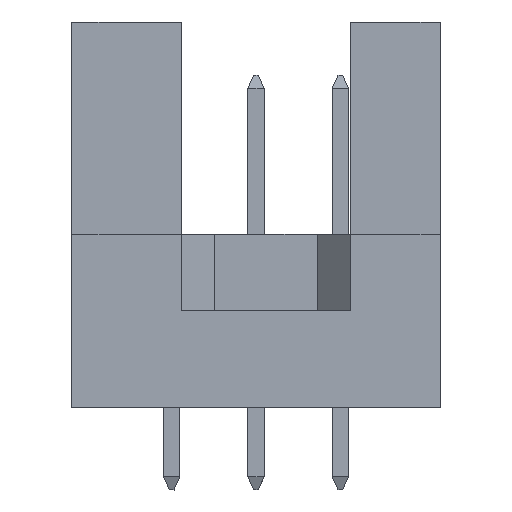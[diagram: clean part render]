
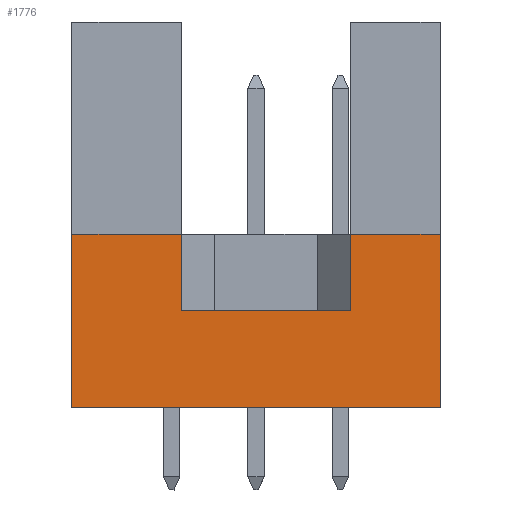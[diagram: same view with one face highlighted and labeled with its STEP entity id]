
A CAD part, left-side view. The second image highlights one B-rep face of the part: STEP entity #1776.
In plain terms, the highlighted planar face has unit normal (-1, 0, 0).
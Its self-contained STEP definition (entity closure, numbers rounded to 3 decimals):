
#225 = LINE ( 'NONE', #3010, #6124 ) ;
#306 = VERTEX_POINT ( 'NONE', #1129 ) ;
#347 = DIRECTION ( 'NONE',  ( 1., 0., 0. ) ) ;
#743 = VERTEX_POINT ( 'NONE', #1926 ) ;
#1129 = CARTESIAN_POINT ( 'NONE',  ( -19.9, 0., 0. ) ) ;
#1169 = DIRECTION ( 'NONE',  ( 0., -1., 0. ) ) ;
#1288 = CARTESIAN_POINT ( 'NONE',  ( -19.9, 11.1, 5.2 ) ) ;
#1315 = CARTESIAN_POINT ( 'NONE',  ( -19.9, 7.79, 2.9 ) ) ;
#1508 = DIRECTION ( 'NONE',  ( 0., 0., 1. ) ) ;
#1773 = VERTEX_POINT ( 'NONE', #5184 ) ;
#1776 = ADVANCED_FACE ( 'NONE', ( #4624 ), #6894, .F. ) ;
#1811 = VERTEX_POINT ( 'NONE', #5438 ) ;
#1817 = DIRECTION ( 'NONE',  ( 0., -1., 0. ) ) ;
#1926 = CARTESIAN_POINT ( 'NONE',  ( -19.9, 7.79, 5.2 ) ) ;
#2096 = CARTESIAN_POINT ( 'NONE',  ( -19.9, 7.79, 2.9 ) ) ;
#2118 = VERTEX_POINT ( 'NONE', #6852 ) ;
#2351 = VECTOR ( 'NONE', #1508, 1000. ) ;
#2395 = VERTEX_POINT ( 'NONE', #2526 ) ;
#2436 = DIRECTION ( 'NONE',  ( 0., 0., 1. ) ) ;
#2471 = LINE ( 'NONE', #3527, #5563 ) ;
#2480 = VECTOR ( 'NONE', #3565, 1000. ) ;
#2526 = CARTESIAN_POINT ( 'NONE',  ( -19.9, 2.71, 5.2 ) ) ;
#2653 = EDGE_LOOP ( 'NONE', ( #4349, #7238, #4545, #3971, #3849, #2853, #6539, #3407 ) ) ;
#2716 = VECTOR ( 'NONE', #2956, 1000. ) ;
#2784 = VECTOR ( 'NONE', #3994, 1000. ) ;
#2853 = ORIENTED_EDGE ( 'NONE', *, *, #4352, .T. ) ;
#2956 = DIRECTION ( 'NONE',  ( 0., 0., 1. ) ) ;
#3010 = CARTESIAN_POINT ( 'NONE',  ( -19.9, 11.1, 5.2 ) ) ;
#3124 = EDGE_CURVE ( 'NONE', #1811, #743, #4549, .T. ) ;
#3391 = CARTESIAN_POINT ( 'NONE',  ( -19.9, 2.71, 2.9 ) ) ;
#3407 = ORIENTED_EDGE ( 'NONE', *, *, #4865, .F. ) ;
#3485 = EDGE_CURVE ( 'NONE', #2395, #2118, #225, .T. ) ;
#3527 = CARTESIAN_POINT ( 'NONE',  ( -19.9, 0., 0. ) ) ;
#3546 = EDGE_CURVE ( 'NONE', #1811, #7051, #6625, .T. ) ;
#3565 = DIRECTION ( 'NONE',  ( 0., -1., 0. ) ) ;
#3849 = ORIENTED_EDGE ( 'NONE', *, *, #4710, .T. ) ;
#3971 = ORIENTED_EDGE ( 'NONE', *, *, #4610, .F. ) ;
#3994 = DIRECTION ( 'NONE',  ( 0., 0., 1. ) ) ;
#4292 = DIRECTION ( 'NONE',  ( 0., -1., 0. ) ) ;
#4300 = CARTESIAN_POINT ( 'NONE',  ( -19.9, 11.1, 0. ) ) ;
#4349 = ORIENTED_EDGE ( 'NONE', *, *, #3546, .F. ) ;
#4352 = EDGE_CURVE ( 'NONE', #306, #2118, #2471, .T. ) ;
#4459 = EDGE_CURVE ( 'NONE', #5923, #743, #6385, .T. ) ;
#4545 = ORIENTED_EDGE ( 'NONE', *, *, #4459, .F. ) ;
#4549 = LINE ( 'NONE', #1315, #2784 ) ;
#4551 = LINE ( 'NONE', #6789, #6636 ) ;
#4610 = EDGE_CURVE ( 'NONE', #1773, #5923, #4858, .T. ) ;
#4624 = FACE_OUTER_BOUND ( 'NONE', #2653, .T. ) ;
#4710 = EDGE_CURVE ( 'NONE', #1773, #306, #4551, .T. ) ;
#4732 = DIRECTION ( 'NONE',  ( 0., 0., -1. ) ) ;
#4739 = LINE ( 'NONE', #6448, #2716 ) ;
#4858 = LINE ( 'NONE', #4300, #2351 ) ;
#4865 = EDGE_CURVE ( 'NONE', #7051, #2395, #4739, .T. ) ;
#5184 = CARTESIAN_POINT ( 'NONE',  ( -19.9, 11.1, 0. ) ) ;
#5438 = CARTESIAN_POINT ( 'NONE',  ( -19.9, 7.79, 2.9 ) ) ;
#5563 = VECTOR ( 'NONE', #2436, 1000. ) ;
#5923 = VERTEX_POINT ( 'NONE', #6578 ) ;
#6124 = VECTOR ( 'NONE', #1817, 1000. ) ;
#6222 = AXIS2_PLACEMENT_3D ( 'NONE', #6478, #347, #4732 ) ;
#6385 = LINE ( 'NONE', #1288, #2480 ) ;
#6448 = CARTESIAN_POINT ( 'NONE',  ( -19.9, 2.71, 2.9 ) ) ;
#6478 = CARTESIAN_POINT ( 'NONE',  ( -19.9, 11.1, 0. ) ) ;
#6539 = ORIENTED_EDGE ( 'NONE', *, *, #3485, .F. ) ;
#6578 = CARTESIAN_POINT ( 'NONE',  ( -19.9, 11.1, 5.2 ) ) ;
#6625 = LINE ( 'NONE', #2096, #6719 ) ;
#6636 = VECTOR ( 'NONE', #1169, 1000. ) ;
#6719 = VECTOR ( 'NONE', #4292, 1000. ) ;
#6789 = CARTESIAN_POINT ( 'NONE',  ( -19.9, 11.1, 0. ) ) ;
#6852 = CARTESIAN_POINT ( 'NONE',  ( -19.9, 0., 5.2 ) ) ;
#6894 = PLANE ( 'NONE',  #6222 ) ;
#7051 = VERTEX_POINT ( 'NONE', #3391 ) ;
#7238 = ORIENTED_EDGE ( 'NONE', *, *, #3124, .T. ) ;
